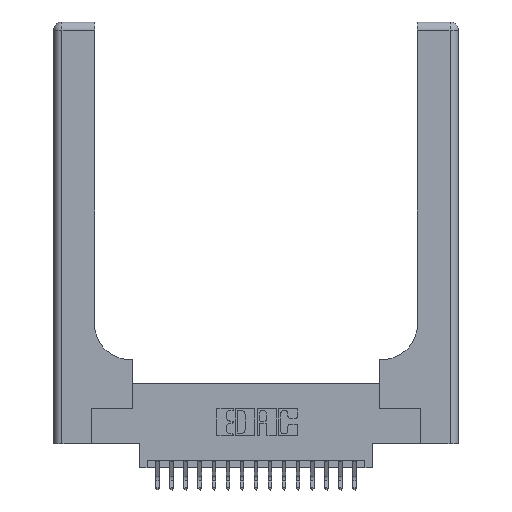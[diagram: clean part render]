
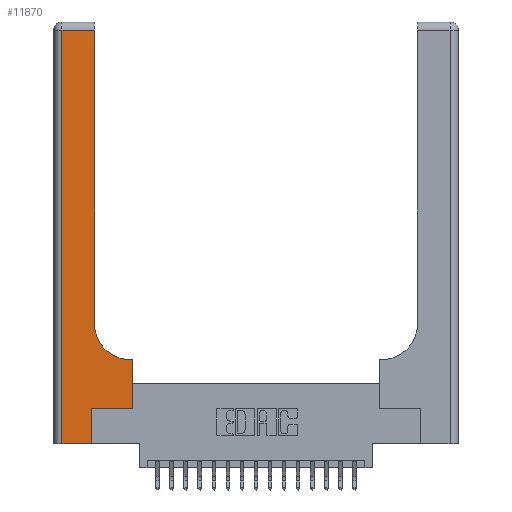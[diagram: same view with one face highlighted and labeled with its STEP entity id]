
A CAD part, top view. The second image highlights one B-rep face of the part: STEP entity #11870.
In plain terms, the highlighted planar face has unit normal (0, 0, 1).
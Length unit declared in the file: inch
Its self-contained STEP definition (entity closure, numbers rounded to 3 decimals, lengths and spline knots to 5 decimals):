
#4 = VERTEX_POINT ( 'NONE', #15622 ) ;
#43 = EDGE_CURVE ( 'NONE', #17677, #2853, #4821, .T. ) ;
#115 = EDGE_LOOP ( 'NONE', ( #12909, #9038, #9174, #10055, #14970, #14639, #17080, #19864, #1924 ) ) ;
#130 = CARTESIAN_POINT ( 'NONE',  ( 0.269, 0., 0.37 ) ) ;
#189 = LINE ( 'NONE', #6838, #6195 ) ;
#499 = CIRCLE ( 'NONE', #14850, 0.25 ) ;
#862 = VERTEX_POINT ( 'NONE', #12015 ) ;
#1129 = LINE ( 'NONE', #4000, #15526 ) ;
#1145 = DIRECTION ( 'NONE',  ( 0., 0., -1. ) ) ;
#1479 = EDGE_CURVE ( 'NONE', #12851, #862, #1129, .T. ) ;
#1803 = CARTESIAN_POINT ( 'NONE',  ( 0.269, 0.25, 0.37 ) ) ;
#1810 = LINE ( 'NONE', #13058, #15207 ) ;
#1924 = ORIENTED_EDGE ( 'NONE', *, *, #18845, .T. ) ;
#2853 = VERTEX_POINT ( 'NONE', #3044 ) ;
#2909 = CARTESIAN_POINT ( 'NONE',  ( 0.269, 0.25, 0.37 ) ) ;
#2979 = EDGE_CURVE ( 'NONE', #862, #4, #1810, .T. ) ;
#3028 = DIRECTION ( 'NONE',  ( 0., 1., 0. ) ) ;
#3044 = CARTESIAN_POINT ( 'NONE',  ( 0.5585, 0.25, 0.37 ) ) ;
#3554 = CARTESIAN_POINT ( 'NONE',  ( 0.06, 0., 0.37 ) ) ;
#3953 = DIRECTION ( 'NONE',  ( 1., 0., 0. ) ) ;
#4000 = CARTESIAN_POINT ( 'NONE',  ( 0.2915, 3., 0.37 ) ) ;
#4497 = PLANE ( 'NONE',  #5673 ) ;
#4582 = DIRECTION ( 'NONE',  ( 1., 0., 0. ) ) ;
#4821 = LINE ( 'NONE', #2909, #13437 ) ;
#4841 = VECTOR ( 'NONE', #3953, 39.37008 ) ;
#5132 = FACE_OUTER_BOUND ( 'NONE', #115, .T. ) ;
#5155 = EDGE_CURVE ( 'NONE', #4, #10509, #19670, .T. ) ;
#5673 = AXIS2_PLACEMENT_3D ( 'NONE', #7580, #18842, #7447 ) ;
#5728 = EDGE_CURVE ( 'NONE', #15659, #20800, #189, .T. ) ;
#6057 = CARTESIAN_POINT ( 'NONE',  ( 0.5415, 0.85, 0.37 ) ) ;
#6166 = DIRECTION ( 'NONE',  ( 0., 1., 0. ) ) ;
#6195 = VECTOR ( 'NONE', #18099, 39.37008 ) ;
#6199 = DIRECTION ( 'NONE',  ( 1., 0., 0. ) ) ;
#6595 = DIRECTION ( 'NONE',  ( -1., 0., 0. ) ) ;
#6838 = CARTESIAN_POINT ( 'NONE',  ( 0.2915, 0.6, 0.37 ) ) ;
#7236 = VECTOR ( 'NONE', #18863, 39.37008 ) ;
#7447 = DIRECTION ( 'NONE',  ( -1., 0., 0. ) ) ;
#7580 = CARTESIAN_POINT ( 'NONE',  ( 0., 3., 0.37 ) ) ;
#7950 = VECTOR ( 'NONE', #12443, 39.37008 ) ;
#8040 = VERTEX_POINT ( 'NONE', #130 ) ;
#8214 = LINE ( 'NONE', #18932, #7950 ) ;
#9038 = ORIENTED_EDGE ( 'NONE', *, *, #2979, .T. ) ;
#9174 = ORIENTED_EDGE ( 'NONE', *, *, #5155, .T. ) ;
#10055 = ORIENTED_EDGE ( 'NONE', *, *, #14808, .T. ) ;
#10509 = VERTEX_POINT ( 'NONE', #3554 ) ;
#10573 = LINE ( 'NONE', #14243, #11869 ) ;
#11048 = CARTESIAN_POINT ( 'NONE',  ( 0.5585, 0.6, 0.37 ) ) ;
#11297 = EDGE_CURVE ( 'NONE', #8040, #17677, #8214, .T. ) ;
#11869 = VECTOR ( 'NONE', #3028, 39.37008 ) ;
#11870 = ADVANCED_FACE ( 'NONE', ( #5132 ), #4497, .F. ) ;
#12015 = CARTESIAN_POINT ( 'NONE',  ( 0.2915, 2.94, 0.37 ) ) ;
#12443 = DIRECTION ( 'NONE',  ( 0., 1., 0. ) ) ;
#12851 = VERTEX_POINT ( 'NONE', #17587 ) ;
#12909 = ORIENTED_EDGE ( 'NONE', *, *, #1479, .T. ) ;
#13058 = CARTESIAN_POINT ( 'NONE',  ( 0., 2.94, 0.37 ) ) ;
#13437 = VECTOR ( 'NONE', #4582, 39.37008 ) ;
#13471 = CARTESIAN_POINT ( 'NONE',  ( 0.5415, 0.6, 0.37 ) ) ;
#14114 = CARTESIAN_POINT ( 'NONE',  ( 0.06, 3., 0.37 ) ) ;
#14160 = EDGE_CURVE ( 'NONE', #2853, #15659, #10573, .T. ) ;
#14243 = CARTESIAN_POINT ( 'NONE',  ( 0.5585, 0.25, 0.37 ) ) ;
#14639 = ORIENTED_EDGE ( 'NONE', *, *, #43, .T. ) ;
#14808 = EDGE_CURVE ( 'NONE', #10509, #8040, #17991, .T. ) ;
#14850 = AXIS2_PLACEMENT_3D ( 'NONE', #6057, #1145, #6199 ) ;
#14970 = ORIENTED_EDGE ( 'NONE', *, *, #11297, .T. ) ;
#15207 = VECTOR ( 'NONE', #6595, 39.37008 ) ;
#15526 = VECTOR ( 'NONE', #6166, 39.37008 ) ;
#15622 = CARTESIAN_POINT ( 'NONE',  ( 0.06, 2.94, 0.37 ) ) ;
#15659 = VERTEX_POINT ( 'NONE', #11048 ) ;
#17080 = ORIENTED_EDGE ( 'NONE', *, *, #14160, .T. ) ;
#17587 = CARTESIAN_POINT ( 'NONE',  ( 0.2915, 0.85, 0.37 ) ) ;
#17677 = VERTEX_POINT ( 'NONE', #1803 ) ;
#17991 = LINE ( 'NONE', #18378, #4841 ) ;
#18099 = DIRECTION ( 'NONE',  ( -1., 0., 0. ) ) ;
#18378 = CARTESIAN_POINT ( 'NONE',  ( 0., 0., 0.37 ) ) ;
#18842 = DIRECTION ( 'NONE',  ( 0., 0., -1. ) ) ;
#18845 = EDGE_CURVE ( 'NONE', #20800, #12851, #499, .T. ) ;
#18863 = DIRECTION ( 'NONE',  ( 0., -1., 0. ) ) ;
#18932 = CARTESIAN_POINT ( 'NONE',  ( 0.269, 0., 0.37 ) ) ;
#19670 = LINE ( 'NONE', #14114, #7236 ) ;
#19864 = ORIENTED_EDGE ( 'NONE', *, *, #5728, .T. ) ;
#20800 = VERTEX_POINT ( 'NONE', #13471 ) ;
